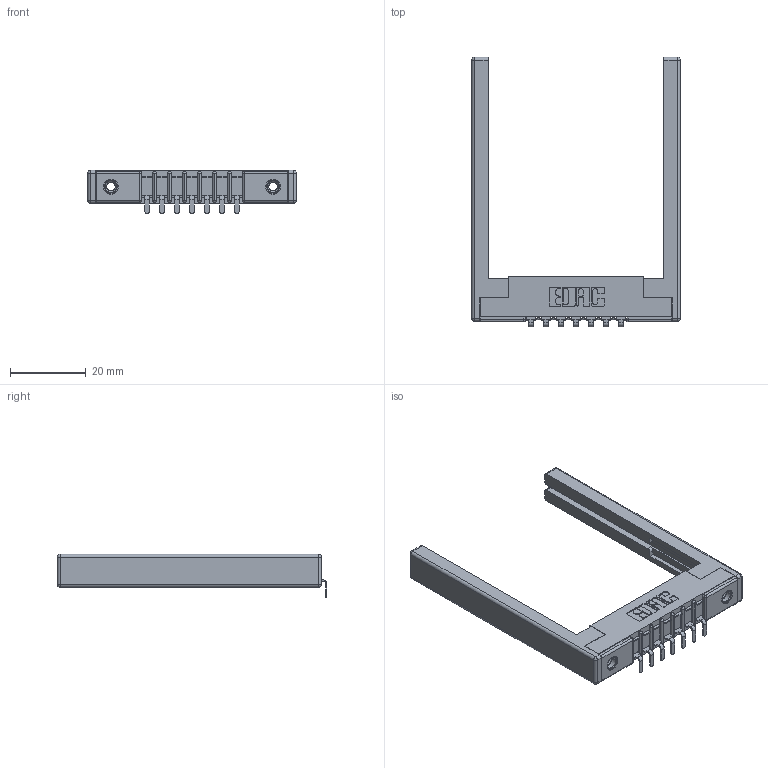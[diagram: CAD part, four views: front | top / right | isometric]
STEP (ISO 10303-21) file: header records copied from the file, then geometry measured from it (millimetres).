
FILE_DESCRIPTION (( 'STEP AP203' ), '1' );
FILE_NAME ('357-007-553-168.STEP', '2019-09-16T17:27:04', ( '' ), ( '' ), 'SwSTEP 2.0', 'SolidWorks 2016', '' );
FILE_SCHEMA (( 'CONFIG_CONTROL_DESIGN' ));
Length unit declared in the file: inch
Products named in the file (5): 345-250-001_345-250-001-102; 307-290-002_553; 307-220-068; 307 Part_.156 Dia Mounting Holes; 357-007-553-168
Assembly tree (12 placements, depth 2):
  357-007-553-168
    307 Part_.156 Dia Mounting Holes
    307-290-002_553  x7
    307-220-068  x2
    345-250-001_345-250-001-102  x2
Bounding box: 55.17 x 71.29 x 11.51 mm (x, y, z)
Volume: 8193 mm3; surface area: 9798.7 mm2
Topology: 12 solids, 12 shells, 826 faces, 2421 edges, 1570 vertices
Faces by surface type: plane 487, cylinder 299, sphere 24, cone 12, torus 4
Entity records: 13929 total; most frequent: CARTESIAN_POINT 2309, ORIENTED_EDGE 2288, DIRECTION 2278, EDGE_CURVE 1144, LINE 856, VECTOR 856, VERTEX_POINT 742, AXIS2_PLACEMENT_3D 711
